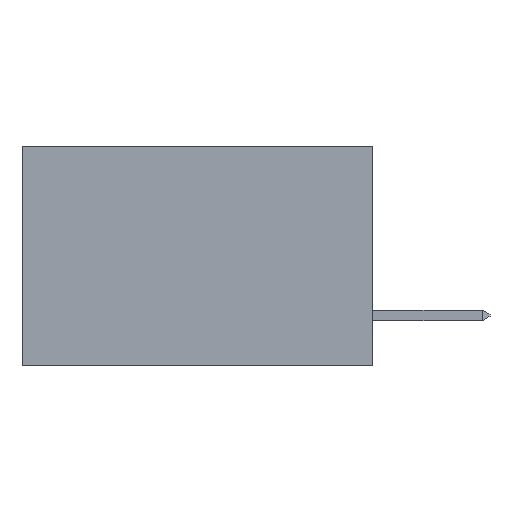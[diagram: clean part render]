
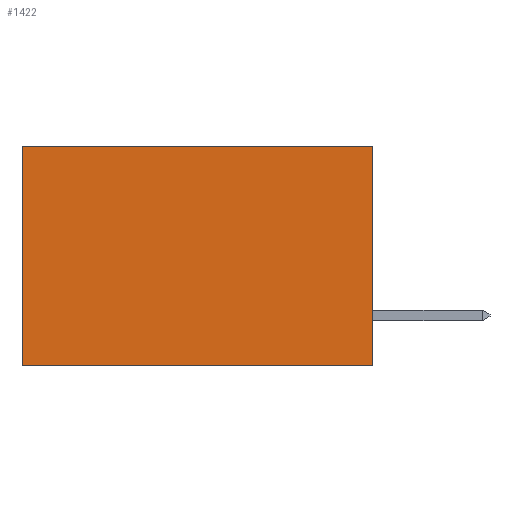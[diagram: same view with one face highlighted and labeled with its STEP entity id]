
A CAD part, left-side view. The second image highlights one B-rep face of the part: STEP entity #1422.
In plain terms, the highlighted planar face has unit normal (-1, 0, 0).
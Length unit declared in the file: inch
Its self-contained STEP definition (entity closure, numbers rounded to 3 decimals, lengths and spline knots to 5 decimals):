
#192 = DIRECTION ( 'NONE',  ( 0., 0., -1. ) ) ;
#247 = VECTOR ( 'NONE', #1140, 39.37008 ) ;
#318 = CARTESIAN_POINT ( 'NONE',  ( 0.277, 0., 0. ) ) ;
#558 = DIRECTION ( 'NONE',  ( 0., 0., -1. ) ) ;
#859 = ORIENTED_EDGE ( 'NONE', *, *, #7788, .T. ) ;
#916 = VECTOR ( 'NONE', #4291, 39.37008 ) ;
#920 = FACE_OUTER_BOUND ( 'NONE', #6971, .T. ) ;
#1140 = DIRECTION ( 'NONE',  ( 0., 1., 0. ) ) ;
#1422 = ADVANCED_FACE ( 'NONE', ( #920 ), #2442, .F. ) ;
#1808 = ORIENTED_EDGE ( 'NONE', *, *, #3001, .F. ) ;
#1911 = EDGE_CURVE ( 'NONE', #5243, #2515, #9844, .T. ) ;
#2151 = ORIENTED_EDGE ( 'NONE', *, *, #8987, .T. ) ;
#2442 = PLANE ( 'NONE',  #3417 ) ;
#2515 = VERTEX_POINT ( 'NONE', #3610 ) ;
#3001 = EDGE_CURVE ( 'NONE', #2515, #6795, #5413, .T. ) ;
#3079 = LINE ( 'NONE', #9929, #916 ) ;
#3193 = DIRECTION ( 'NONE',  ( 0., 1., 0. ) ) ;
#3331 = VERTEX_POINT ( 'NONE', #3982 ) ;
#3400 = ORIENTED_EDGE ( 'NONE', *, *, #1911, .F. ) ;
#3417 = AXIS2_PLACEMENT_3D ( 'NONE', #6706, #6688, #558 ) ;
#3437 = CARTESIAN_POINT ( 'NONE',  ( 0.277, 0., -0.37 ) ) ;
#3610 = CARTESIAN_POINT ( 'NONE',  ( 0.277, 0., -0.37 ) ) ;
#3982 = CARTESIAN_POINT ( 'NONE',  ( 0.277, 0.59, 0. ) ) ;
#4291 = DIRECTION ( 'NONE',  ( 0., 0., -1. ) ) ;
#4580 = CARTESIAN_POINT ( 'NONE',  ( 0.277, 0.59, -0.37 ) ) ;
#5243 = VERTEX_POINT ( 'NONE', #8212 ) ;
#5413 = LINE ( 'NONE', #3437, #9697 ) ;
#6498 = CARTESIAN_POINT ( 'NONE',  ( 0.277, 0., -0.37 ) ) ;
#6686 = LINE ( 'NONE', #318, #247 ) ;
#6688 = DIRECTION ( 'NONE',  ( 1., 0., 0. ) ) ;
#6706 = CARTESIAN_POINT ( 'NONE',  ( 0.277, 0., -0.37 ) ) ;
#6795 = VERTEX_POINT ( 'NONE', #4580 ) ;
#6971 = EDGE_LOOP ( 'NONE', ( #859, #1808, #3400, #2151 ) ) ;
#7788 = EDGE_CURVE ( 'NONE', #3331, #6795, #3079, .T. ) ;
#8212 = CARTESIAN_POINT ( 'NONE',  ( 0.277, 0., 0. ) ) ;
#8987 = EDGE_CURVE ( 'NONE', #5243, #3331, #6686, .T. ) ;
#9600 = VECTOR ( 'NONE', #192, 39.37008 ) ;
#9697 = VECTOR ( 'NONE', #3193, 39.37008 ) ;
#9844 = LINE ( 'NONE', #6498, #9600 ) ;
#9929 = CARTESIAN_POINT ( 'NONE',  ( 0.277, 0.59, -0.37 ) ) ;
